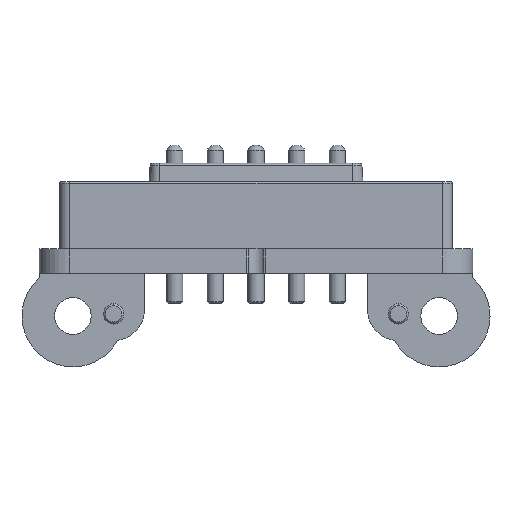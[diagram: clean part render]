
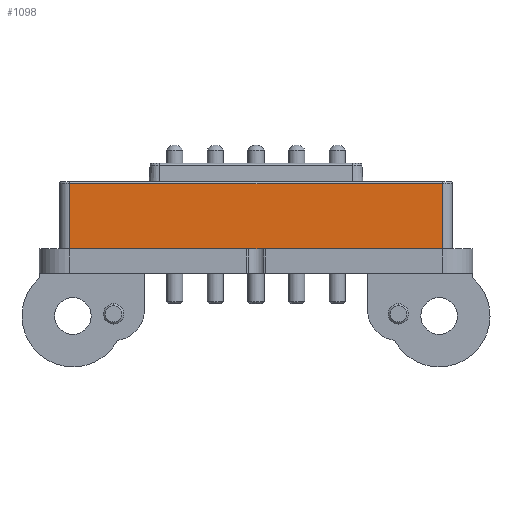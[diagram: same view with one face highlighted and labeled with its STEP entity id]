
A CAD part, front view. The second image highlights one B-rep face of the part: STEP entity #1098.
In plain terms, the highlighted planar face has unit normal (0, -1, 0).
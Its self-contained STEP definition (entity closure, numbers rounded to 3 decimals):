
#864 = LINE ( 'NONE', #9142, #14438 ) ;
#1050 = DIRECTION ( 'NONE',  ( 1., 0., 0. ) ) ;
#1098 = ADVANCED_FACE ( 'NONE', ( #9435 ), #4672, .F. ) ;
#1112 = VERTEX_POINT ( 'NONE', #2612 ) ;
#1213 = VECTOR ( 'NONE', #8224, 1000. ) ;
#1539 = DIRECTION ( 'NONE',  ( 0., 1., 0. ) ) ;
#1605 = ORIENTED_EDGE ( 'NONE', *, *, #10644, .T. ) ;
#2300 = ORIENTED_EDGE ( 'NONE', *, *, #14748, .T. ) ;
#2612 = CARTESIAN_POINT ( 'NONE',  ( -9.15, -2.5, -0.1 ) ) ;
#2659 = DIRECTION ( 'NONE',  ( 0., 0., 1. ) ) ;
#3458 = CARTESIAN_POINT ( 'NONE',  ( -9.15, -2.5, -0.1 ) ) ;
#4196 = CARTESIAN_POINT ( 'NONE',  ( 9.15, -2.5, -3.3 ) ) ;
#4672 = PLANE ( 'NONE',  #14816 ) ;
#5033 = LINE ( 'NONE', #7500, #8897 ) ;
#5615 = DIRECTION ( 'NONE',  ( -1., 0., 0. ) ) ;
#6174 = EDGE_CURVE ( 'NONE', #12109, #12427, #5033, .T. ) ;
#6210 = DIRECTION ( 'NONE',  ( 1., 0., 0. ) ) ;
#6667 = ORIENTED_EDGE ( 'NONE', *, *, #8361, .T. ) ;
#6940 = EDGE_LOOP ( 'NONE', ( #6667, #2300, #8204, #1605 ) ) ;
#7127 = VERTEX_POINT ( 'NONE', #8902 ) ;
#7285 = VECTOR ( 'NONE', #1050, 1000. ) ;
#7500 = CARTESIAN_POINT ( 'NONE',  ( 9.15, -2.5, -3.3 ) ) ;
#8204 = ORIENTED_EDGE ( 'NONE', *, *, #6174, .T. ) ;
#8224 = DIRECTION ( 'NONE',  ( 0., 0., -1. ) ) ;
#8361 = EDGE_CURVE ( 'NONE', #1112, #7127, #10010, .T. ) ;
#8897 = VECTOR ( 'NONE', #2659, 1000. ) ;
#8902 = CARTESIAN_POINT ( 'NONE',  ( -9.15, -2.5, -3.3 ) ) ;
#9142 = CARTESIAN_POINT ( 'NONE',  ( 9.15, -2.5, -0.1 ) ) ;
#9435 = FACE_OUTER_BOUND ( 'NONE', #6940, .T. ) ;
#9731 = CARTESIAN_POINT ( 'NONE',  ( 0., -2.5, -1.7 ) ) ;
#10010 = LINE ( 'NONE', #3458, #1213 ) ;
#10644 = EDGE_CURVE ( 'NONE', #12427, #1112, #864, .T. ) ;
#12109 = VERTEX_POINT ( 'NONE', #4196 ) ;
#12427 = VERTEX_POINT ( 'NONE', #14322 ) ;
#14027 = LINE ( 'NONE', #15092, #7285 ) ;
#14322 = CARTESIAN_POINT ( 'NONE',  ( 9.15, -2.5, -0.1 ) ) ;
#14438 = VECTOR ( 'NONE', #5615, 1000. ) ;
#14748 = EDGE_CURVE ( 'NONE', #7127, #12109, #14027, .T. ) ;
#14816 = AXIS2_PLACEMENT_3D ( 'NONE', #9731, #1539, #6210 ) ;
#15092 = CARTESIAN_POINT ( 'NONE',  ( -9.15, -2.5, -3.3 ) ) ;
